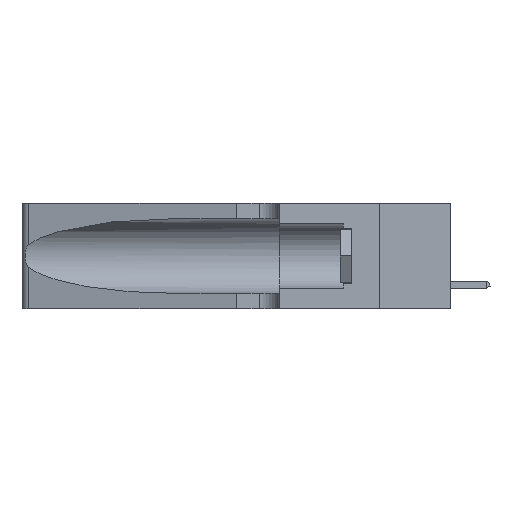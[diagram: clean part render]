
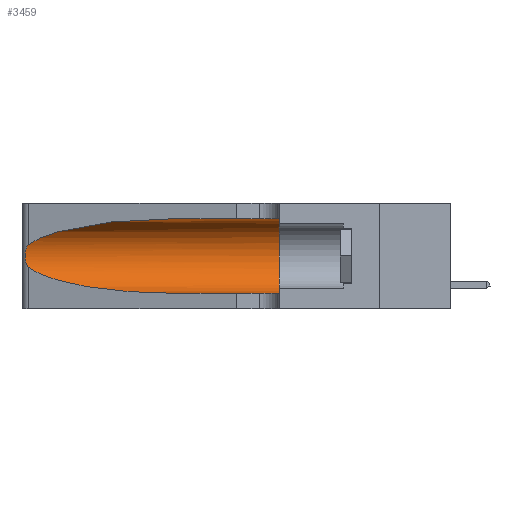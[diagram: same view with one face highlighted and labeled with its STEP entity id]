
A CAD part, left-side view. The second image highlights one B-rep face of the part: STEP entity #3459.
In plain terms, the highlighted cylindrical face has radius 3.308 mm (diameter 6.617 mm), a partial arc.
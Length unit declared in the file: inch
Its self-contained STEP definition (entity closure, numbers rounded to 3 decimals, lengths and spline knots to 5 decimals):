
#273 = EDGE_CURVE ( 'NONE', #23877, #7061, #7499, .T. ) ;
#525 = LINE ( 'NONE', #9162, #5398 ) ;
#1130 = CARTESIAN_POINT ( 'NONE',  ( 0.1305, 0.72297, 0.31525 ) ) ;
#1305 = EDGE_LOOP ( 'NONE', ( #16220, #11663, #13907, #23872, #5459, #15040 ) ) ;
#3459 = ADVANCED_FACE ( 'NONE', ( #6905 ), #26414, .F. ) ;
#3815 = EDGE_CURVE ( 'NONE', #23877, #16667, #23796, .T. ) ;
#4480 = CARTESIAN_POINT ( 'NONE',  ( 0.25487, 1.22718, 0.14631 ) ) ;
#4821 = CARTESIAN_POINT ( 'NONE',  ( 0.1305, 0.72297, 0.05475 ) ) ;
#5398 = VECTOR ( 'NONE', #9034, 39.37008 ) ;
#5459 = ORIENTED_EDGE ( 'NONE', *, *, #5502, .F. ) ;
#5485 = CARTESIAN_POINT ( 'NONE',  ( 0.25639, 1.23186, 0.15144 ) ) ;
#5502 = EDGE_CURVE ( 'NONE', #16667, #28570, #32071, .T. ) ;
#6905 = FACE_OUTER_BOUND ( 'NONE', #1305, .T. ) ;
#6941 = EDGE_CURVE ( 'NONE', #7061, #19079, #22259, .T. ) ;
#7061 = VERTEX_POINT ( 'NONE', #23880 ) ;
#7349 = CARTESIAN_POINT ( 'NONE',  ( 0.18966, 0.96281, 0.05475 ) ) ;
#7499 =( BOUNDED_CURVE ( )  B_SPLINE_CURVE ( 3, ( #19254, #8214, #8091, #36695 ),
 .UNSPECIFIED., .F., .F. ) 
 B_SPLINE_CURVE_WITH_KNOTS ( ( 4, 4 ),
 ( 1.5708, 2.84003 ),
 .UNSPECIFIED. ) 
 CURVE ( )  GEOMETRIC_REPRESENTATION_ITEM ( )  RATIONAL_B_SPLINE_CURVE ( ( 1., 0.87, 0.87, 1. ) ) 
 REPRESENTATION_ITEM ( '' )  );
#8091 = CARTESIAN_POINT ( 'NONE',  ( 0.2373, 1.15595, 0.28018 ) ) ;
#8214 = CARTESIAN_POINT ( 'NONE',  ( 0.18966, 0.96281, 0.31525 ) ) ;
#9034 = DIRECTION ( 'NONE',  ( 0., -1., 0. ) ) ;
#9162 = CARTESIAN_POINT ( 'NONE',  ( 0.1305, 1.61858, 0.05475 ) ) ;
#10130 = DIRECTION ( 'NONE',  ( 0., 0., 1. ) ) ;
#11093 = CARTESIAN_POINT ( 'NONE',  ( 0.26075, 1.23896, 0.178 ) ) ;
#11654 = CARTESIAN_POINT ( 'NONE',  ( 0.1305, 0.72297, 0.05475 ) ) ;
#11663 = ORIENTED_EDGE ( 'NONE', *, *, #6941, .T. ) ;
#13556 = CARTESIAN_POINT ( 'NONE',  ( 0.2373, 1.15595, 0.08982 ) ) ;
#13907 = ORIENTED_EDGE ( 'NONE', *, *, #14950, .T. ) ;
#13964 = CARTESIAN_POINT ( 'NONE',  ( 0.25856, 1.23593, 0.16098 ) ) ;
#14950 = EDGE_CURVE ( 'NONE', #19079, #26159, #15668, .T. ) ;
#15040 = ORIENTED_EDGE ( 'NONE', *, *, #3815, .F. ) ;
#15668 =( BOUNDED_CURVE ( )  B_SPLINE_CURVE ( 3, ( #21726, #13556, #7349, #4821 ),
 .UNSPECIFIED., .F., .F. ) 
 B_SPLINE_CURVE_WITH_KNOTS ( ( 4, 4 ),
 ( 3.44316, 4.71239 ),
 .UNSPECIFIED. ) 
 CURVE ( )  GEOMETRIC_REPRESENTATION_ITEM ( )  RATIONAL_B_SPLINE_CURVE ( ( 1., 0.87, 0.87, 1. ) ) 
 REPRESENTATION_ITEM ( '' )  );
#16220 = ORIENTED_EDGE ( 'NONE', *, *, #273, .T. ) ;
#16386 = CARTESIAN_POINT ( 'NONE',  ( 0.1305, 1.61858, 0.185 ) ) ;
#16550 = CARTESIAN_POINT ( 'NONE',  ( 0.25487, 1.22718, 0.22369 ) ) ;
#16667 = VERTEX_POINT ( 'NONE', #17669 ) ;
#16798 = CARTESIAN_POINT ( 'NONE',  ( 0.25555, 1.22993, 0.14849 ) ) ;
#17669 = CARTESIAN_POINT ( 'NONE',  ( 0.1305, 0.35, 0.31525 ) ) ;
#18295 = EDGE_CURVE ( 'NONE', #26159, #28570, #525, .T. ) ;
#19079 = VERTEX_POINT ( 'NONE', #4480 ) ;
#19254 = CARTESIAN_POINT ( 'NONE',  ( 0.1305, 0.72297, 0.31525 ) ) ;
#19401 = CARTESIAN_POINT ( 'NONE',  ( 0.25787, 1.23484, 0.2124 ) ) ;
#19730 = DIRECTION ( 'NONE',  ( 0., -1., 0. ) ) ;
#19857 = DIRECTION ( 'NONE',  ( 0., 0., -1. ) ) ;
#21297 = CARTESIAN_POINT ( 'NONE',  ( 0.1305, 0.35, 0.185 ) ) ;
#21463 = AXIS2_PLACEMENT_3D ( 'NONE', #16386, #19730, #19857 ) ;
#21660 = DIRECTION ( 'NONE',  ( 0., 1., 0. ) ) ;
#21726 = CARTESIAN_POINT ( 'NONE',  ( 0.25487, 1.22718, 0.14631 ) ) ;
#22219 = AXIS2_PLACEMENT_3D ( 'NONE', #21297, #21660, #10130 ) ;
#22259 = B_SPLINE_CURVE_WITH_KNOTS ( 'NONE', 3,
 ( #16550, #22753, #22630, #19401, #36839, #33980, #28101, #11093, #30957, #13964, #33848, #5485, #16798, #25358 ),
 .UNSPECIFIED., .F., .F.,
 ( 4, 2, 2, 2, 2, 2, 4 ),
 ( 0., 0.00027, 0.00053, 0.00107, 0.0016, 0.00187, 0.00214 ),
 .UNSPECIFIED. ) ;
#22630 = CARTESIAN_POINT ( 'NONE',  ( 0.25639, 1.23184, 0.21858 ) ) ;
#22753 = CARTESIAN_POINT ( 'NONE',  ( 0.25555, 1.22994, 0.2215 ) ) ;
#23796 = LINE ( 'NONE', #33411, #35853 ) ;
#23872 = ORIENTED_EDGE ( 'NONE', *, *, #18295, .T. ) ;
#23877 = VERTEX_POINT ( 'NONE', #1130 ) ;
#23880 = CARTESIAN_POINT ( 'NONE',  ( 0.25487, 1.22718, 0.22369 ) ) ;
#25358 = CARTESIAN_POINT ( 'NONE',  ( 0.25487, 1.22718, 0.14631 ) ) ;
#26159 = VERTEX_POINT ( 'NONE', #11654 ) ;
#26414 = CYLINDRICAL_SURFACE ( 'NONE', #21463, 0.13025 ) ;
#28101 = CARTESIAN_POINT ( 'NONE',  ( 0.26075, 1.23896, 0.19203 ) ) ;
#28570 = VERTEX_POINT ( 'NONE', #33866 ) ;
#30957 = CARTESIAN_POINT ( 'NONE',  ( 0.26017, 1.23833, 0.17102 ) ) ;
#32071 = CIRCLE ( 'NONE', #22219, 0.13025 ) ;
#33173 = DIRECTION ( 'NONE',  ( 0., -1., 0. ) ) ;
#33411 = CARTESIAN_POINT ( 'NONE',  ( 0.1305, 1.61858, 0.31525 ) ) ;
#33848 = CARTESIAN_POINT ( 'NONE',  ( 0.25789, 1.23486, 0.15765 ) ) ;
#33866 = CARTESIAN_POINT ( 'NONE',  ( 0.1305, 0.35, 0.05475 ) ) ;
#33980 = CARTESIAN_POINT ( 'NONE',  ( 0.26018, 1.23835, 0.19895 ) ) ;
#35853 = VECTOR ( 'NONE', #33173, 39.37008 ) ;
#36695 = CARTESIAN_POINT ( 'NONE',  ( 0.25487, 1.22718, 0.22369 ) ) ;
#36839 = CARTESIAN_POINT ( 'NONE',  ( 0.25854, 1.2359, 0.20912 ) ) ;
